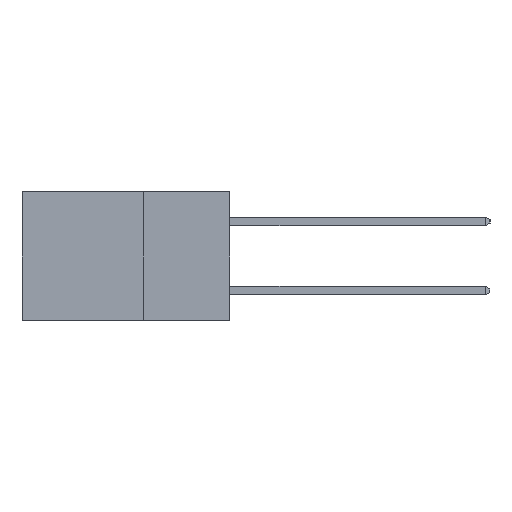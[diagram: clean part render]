
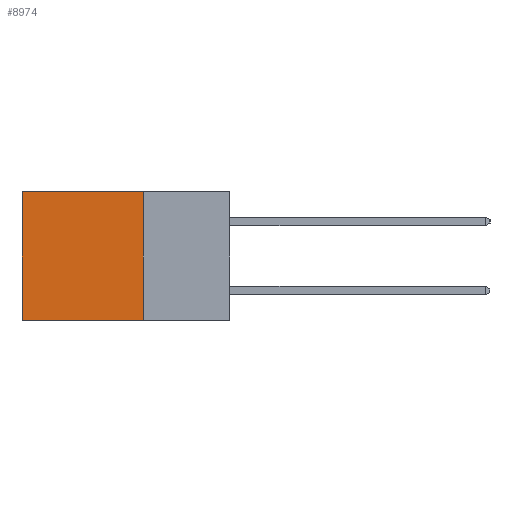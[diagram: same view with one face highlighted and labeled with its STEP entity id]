
A CAD part, left-side view. The second image highlights one B-rep face of the part: STEP entity #8974.
In plain terms, the highlighted planar face has unit normal (-1, 0, 0).
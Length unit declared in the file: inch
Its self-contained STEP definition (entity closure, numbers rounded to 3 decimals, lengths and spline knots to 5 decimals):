
#118 = DIRECTION ( 'NONE',  ( 0., 1., 0. ) ) ;
#198 = CARTESIAN_POINT ( 'NONE',  ( 0.2615, 0.25, 0. ) ) ;
#2559 = EDGE_CURVE ( 'NONE', #9882, #5951, #9060, .T. ) ;
#4117 = DIRECTION ( 'NONE',  ( 0., 0., -1. ) ) ;
#4136 = DIRECTION ( 'NONE',  ( 1., 0., 0. ) ) ;
#4197 = PLANE ( 'NONE',  #18437 ) ;
#4522 = CARTESIAN_POINT ( 'NONE',  ( 0.2615, 0.25, -0.37 ) ) ;
#4743 = ORIENTED_EDGE ( 'NONE', *, *, #2559, .F. ) ;
#4751 = EDGE_CURVE ( 'NONE', #6010, #9882, #16189, .T. ) ;
#5951 = VERTEX_POINT ( 'NONE', #18044 ) ;
#6010 = VERTEX_POINT ( 'NONE', #17599 ) ;
#7174 = LINE ( 'NONE', #19246, #20734 ) ;
#8210 = LINE ( 'NONE', #198, #17293 ) ;
#8485 = VERTEX_POINT ( 'NONE', #15576 ) ;
#8974 = ADVANCED_FACE ( 'NONE', ( #12009 ), #4197, .F. ) ;
#9060 = LINE ( 'NONE', #14741, #17583 ) ;
#9198 = EDGE_CURVE ( 'NONE', #6010, #8485, #8210, .T. ) ;
#9821 = ORIENTED_EDGE ( 'NONE', *, *, #4751, .F. ) ;
#9882 = VERTEX_POINT ( 'NONE', #21750 ) ;
#10024 = ORIENTED_EDGE ( 'NONE', *, *, #9198, .T. ) ;
#10274 = EDGE_LOOP ( 'NONE', ( #11565, #4743, #9821, #10024 ) ) ;
#10918 = DIRECTION ( 'NONE',  ( 0., 0., -1. ) ) ;
#11565 = ORIENTED_EDGE ( 'NONE', *, *, #15420, .T. ) ;
#12009 = FACE_OUTER_BOUND ( 'NONE', #10274, .T. ) ;
#13100 = DIRECTION ( 'NONE',  ( 0., 0., -1. ) ) ;
#14741 = CARTESIAN_POINT ( 'NONE',  ( 0.2615, 0.25, -0.37 ) ) ;
#15420 = EDGE_CURVE ( 'NONE', #8485, #5951, #7174, .T. ) ;
#15576 = CARTESIAN_POINT ( 'NONE',  ( 0.2615, 0.6, 0. ) ) ;
#16189 = LINE ( 'NONE', #18302, #20075 ) ;
#17293 = VECTOR ( 'NONE', #118, 39.37008 ) ;
#17583 = VECTOR ( 'NONE', #18183, 39.37008 ) ;
#17599 = CARTESIAN_POINT ( 'NONE',  ( 0.2615, 0.25, 0. ) ) ;
#18044 = CARTESIAN_POINT ( 'NONE',  ( 0.2615, 0.6, -0.37 ) ) ;
#18183 = DIRECTION ( 'NONE',  ( 0., 1., 0. ) ) ;
#18302 = CARTESIAN_POINT ( 'NONE',  ( 0.2615, 0.25, -0.37 ) ) ;
#18437 = AXIS2_PLACEMENT_3D ( 'NONE', #4522, #4136, #4117 ) ;
#19246 = CARTESIAN_POINT ( 'NONE',  ( 0.2615, 0.6, -0.37 ) ) ;
#20075 = VECTOR ( 'NONE', #13100, 39.37008 ) ;
#20734 = VECTOR ( 'NONE', #10918, 39.37008 ) ;
#21750 = CARTESIAN_POINT ( 'NONE',  ( 0.2615, 0.25, -0.37 ) ) ;
